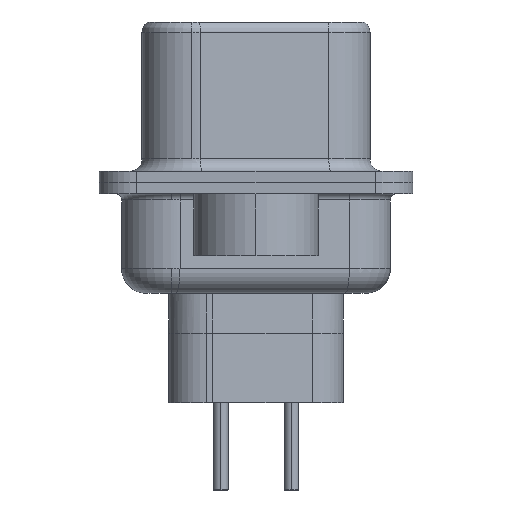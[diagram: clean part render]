
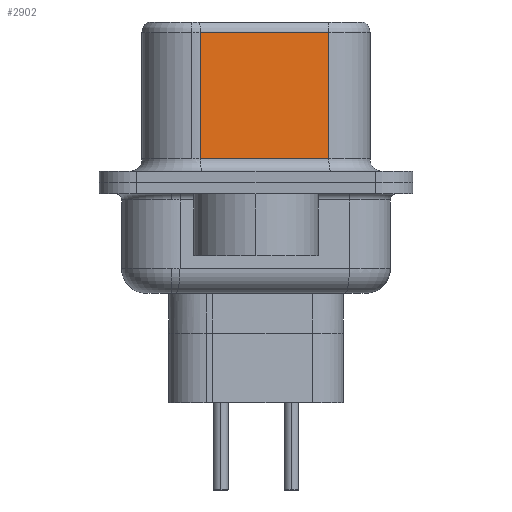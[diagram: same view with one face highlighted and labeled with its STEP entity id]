
A CAD part, left-side view. The second image highlights one B-rep face of the part: STEP entity #2902.
In plain terms, the highlighted planar face has unit normal (-0.985, -0.174, 0).
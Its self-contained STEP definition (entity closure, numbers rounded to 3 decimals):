
#149 = ORIENTED_EDGE ( 'NONE', *, *, #17275, .T. ) ;
#199 = LINE ( 'NONE', #15142, #2581 ) ;
#949 = VERTEX_POINT ( 'NONE', #2884 ) ;
#1097 = VERTEX_POINT ( 'NONE', #4716 ) ;
#1606 = ORIENTED_EDGE ( 'NONE', *, *, #8736, .T. ) ;
#2581 = VECTOR ( 'NONE', #14952, 1000. ) ;
#2884 = CARTESIAN_POINT ( 'NONE',  ( 4.575, -2.927, 6.02 ) ) ;
#2902 = ADVANCED_FACE ( 'NONE', ( #18938 ), #18753, .F. ) ;
#3296 = CARTESIAN_POINT ( 'NONE',  ( 3.665, 2.233, 6.02 ) ) ;
#3550 = LINE ( 'NONE', #16802, #8569 ) ;
#3797 = CARTESIAN_POINT ( 'NONE',  ( 3.665, 2.233, 6.52 ) ) ;
#4333 = CARTESIAN_POINT ( 'NONE',  ( 4.575, -2.927, 0.95 ) ) ;
#4716 = CARTESIAN_POINT ( 'NONE',  ( 3.665, 2.233, 0.95 ) ) ;
#6238 = VECTOR ( 'NONE', #17281, 1000. ) ;
#6734 = VERTEX_POINT ( 'NONE', #4333 ) ;
#8569 = VECTOR ( 'NONE', #18285, 1000. ) ;
#8736 = EDGE_CURVE ( 'NONE', #18119, #1097, #13816, .T. ) ;
#9294 = ORIENTED_EDGE ( 'NONE', *, *, #12256, .T. ) ;
#9556 = VECTOR ( 'NONE', #17259, 1000. ) ;
#10599 = ORIENTED_EDGE ( 'NONE', *, *, #14400, .F. ) ;
#10945 = EDGE_LOOP ( 'NONE', ( #10599, #9294, #1606, #149 ) ) ;
#11416 = DIRECTION ( 'NONE',  ( -0.174, 0.985, 0. ) ) ;
#12256 = EDGE_CURVE ( 'NONE', #949, #18119, #14224, .T. ) ;
#13816 = LINE ( 'NONE', #3797, #9556 ) ;
#14224 = LINE ( 'NONE', #18575, #6238 ) ;
#14400 = EDGE_CURVE ( 'NONE', #949, #6734, #199, .T. ) ;
#14952 = DIRECTION ( 'NONE',  ( 0., 0., -1. ) ) ;
#15142 = CARTESIAN_POINT ( 'NONE',  ( 4.575, -2.927, 6.52 ) ) ;
#15567 = AXIS2_PLACEMENT_3D ( 'NONE', #17459, #18849, #11416 ) ;
#16802 = CARTESIAN_POINT ( 'NONE',  ( 4.575, -2.927, 0.95 ) ) ;
#17259 = DIRECTION ( 'NONE',  ( 0., 0., -1. ) ) ;
#17275 = EDGE_CURVE ( 'NONE', #1097, #6734, #3550, .T. ) ;
#17281 = DIRECTION ( 'NONE',  ( -0.174, 0.985, 0. ) ) ;
#17459 = CARTESIAN_POINT ( 'NONE',  ( 4.575, -2.927, 6.52 ) ) ;
#18119 = VERTEX_POINT ( 'NONE', #3296 ) ;
#18285 = DIRECTION ( 'NONE',  ( 0.174, -0.985, 0. ) ) ;
#18575 = CARTESIAN_POINT ( 'NONE',  ( 4.575, -2.927, 6.02 ) ) ;
#18753 = PLANE ( 'NONE',  #15567 ) ;
#18849 = DIRECTION ( 'NONE',  ( 0.985, 0.174, 0. ) ) ;
#18938 = FACE_OUTER_BOUND ( 'NONE', #10945, .T. ) ;
